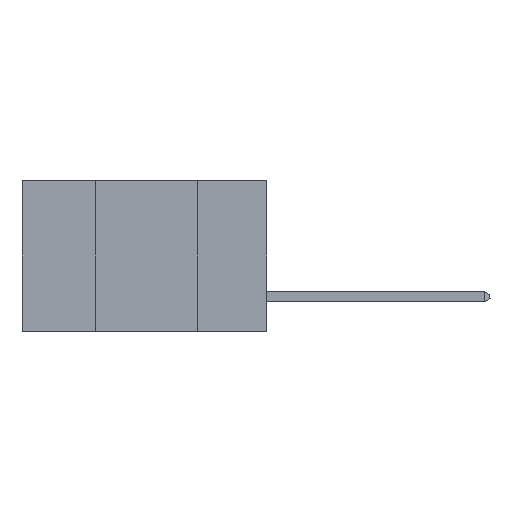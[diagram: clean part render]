
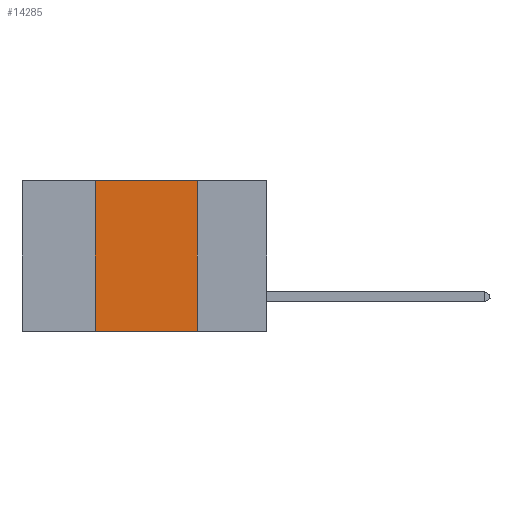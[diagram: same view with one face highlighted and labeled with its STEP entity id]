
A CAD part, left-side view. The second image highlights one B-rep face of the part: STEP entity #14285.
In plain terms, the highlighted planar face has unit normal (-1, 0, 0).
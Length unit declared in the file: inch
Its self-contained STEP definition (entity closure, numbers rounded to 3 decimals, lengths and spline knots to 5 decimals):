
#877 = DIRECTION ( 'NONE',  ( 0., -1., 0. ) ) ;
#1534 = CARTESIAN_POINT ( 'NONE',  ( 0., 0.42, 0. ) ) ;
#1652 = LINE ( 'NONE', #2368, #12707 ) ;
#2368 = CARTESIAN_POINT ( 'NONE',  ( 0., 0.6, 0. ) ) ;
#2447 = VECTOR ( 'NONE', #877, 39.37008 ) ;
#3219 = EDGE_CURVE ( 'NONE', #10357, #18504, #13988, .T. ) ;
#3320 = ORIENTED_EDGE ( 'NONE', *, *, #14004, .F. ) ;
#3751 = DIRECTION ( 'NONE',  ( 1., 0., 0. ) ) ;
#5098 = VECTOR ( 'NONE', #10260, 39.37008 ) ;
#5132 = CARTESIAN_POINT ( 'NONE',  ( 0., 0.6, 0. ) ) ;
#5329 = VECTOR ( 'NONE', #12243, 39.37008 ) ;
#5508 = EDGE_LOOP ( 'NONE', ( #11784, #16821, #3320, #17849 ) ) ;
#7382 = LINE ( 'NONE', #9009, #5329 ) ;
#9009 = CARTESIAN_POINT ( 'NONE',  ( 0., 0.17, 0. ) ) ;
#9730 = EDGE_CURVE ( 'NONE', #11511, #14598, #1652, .T. ) ;
#10260 = DIRECTION ( 'NONE',  ( 0., 0., 1. ) ) ;
#10357 = VERTEX_POINT ( 'NONE', #11046 ) ;
#11046 = CARTESIAN_POINT ( 'NONE',  ( 0., 0.42, -0.37 ) ) ;
#11057 = DIRECTION ( 'NONE',  ( 0., 0., -1. ) ) ;
#11511 = VERTEX_POINT ( 'NONE', #15521 ) ;
#11781 = CARTESIAN_POINT ( 'NONE',  ( 0., 0.17, 0. ) ) ;
#11784 = ORIENTED_EDGE ( 'NONE', *, *, #13893, .F. ) ;
#11879 = LINE ( 'NONE', #1534, #5098 ) ;
#12243 = DIRECTION ( 'NONE',  ( 0., 0., -1. ) ) ;
#12707 = VECTOR ( 'NONE', #13928, 39.37008 ) ;
#12725 = FACE_OUTER_BOUND ( 'NONE', #5508, .T. ) ;
#13401 = AXIS2_PLACEMENT_3D ( 'NONE', #5132, #3751, #11057 ) ;
#13893 = EDGE_CURVE ( 'NONE', #14598, #18504, #7382, .T. ) ;
#13928 = DIRECTION ( 'NONE',  ( 0., -1., 0. ) ) ;
#13988 = LINE ( 'NONE', #18263, #2447 ) ;
#14004 = EDGE_CURVE ( 'NONE', #10357, #11511, #11879, .T. ) ;
#14285 = ADVANCED_FACE ( 'NONE', ( #12725 ), #15380, .F. ) ;
#14598 = VERTEX_POINT ( 'NONE', #11781 ) ;
#15380 = PLANE ( 'NONE',  #13401 ) ;
#15521 = CARTESIAN_POINT ( 'NONE',  ( 0., 0.42, 0. ) ) ;
#16821 = ORIENTED_EDGE ( 'NONE', *, *, #9730, .F. ) ;
#17140 = CARTESIAN_POINT ( 'NONE',  ( 0., 0.17, -0.37 ) ) ;
#17849 = ORIENTED_EDGE ( 'NONE', *, *, #3219, .T. ) ;
#18263 = CARTESIAN_POINT ( 'NONE',  ( 0., 0.6, -0.37 ) ) ;
#18504 = VERTEX_POINT ( 'NONE', #17140 ) ;
